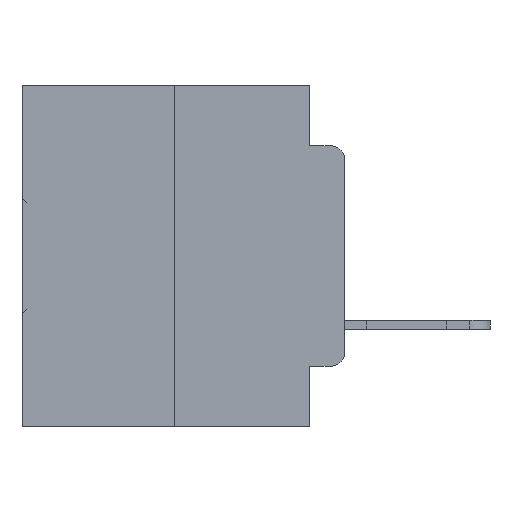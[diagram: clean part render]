
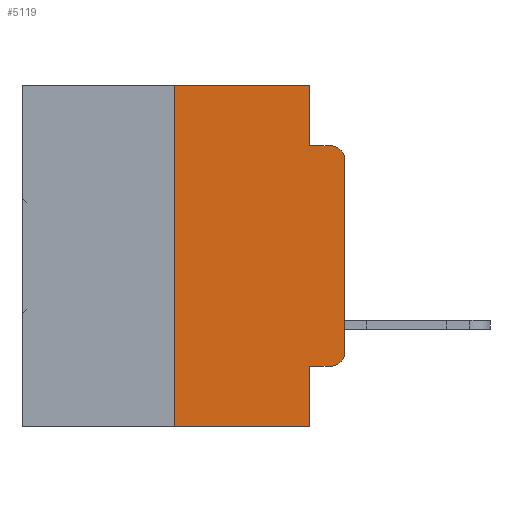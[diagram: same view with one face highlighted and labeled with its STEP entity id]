
A CAD part, left-side view. The second image highlights one B-rep face of the part: STEP entity #5119.
In plain terms, the highlighted planar face has unit normal (-1, 0, 0).
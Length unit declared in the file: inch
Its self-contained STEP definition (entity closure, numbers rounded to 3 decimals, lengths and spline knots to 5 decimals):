
#803 = EDGE_CURVE ( 'NONE', #9963, #8010, #15396, .T. ) ;
#901 = LINE ( 'NONE', #18941, #27302 ) ;
#1038 = VECTOR ( 'NONE', #20745, 39.37008 ) ;
#1166 = CARTESIAN_POINT ( 'NONE',  ( 0., 0.02, -0.1085 ) ) ;
#1177 = ORIENTED_EDGE ( 'NONE', *, *, #20023, .F. ) ;
#1184 = LINE ( 'NONE', #7125, #21236 ) ;
#1892 = ORIENTED_EDGE ( 'NONE', *, *, #803, .T. ) ;
#1928 = DIRECTION ( 'NONE',  ( 0., 0., 1. ) ) ;
#2142 = VECTOR ( 'NONE', #24793, 39.37008 ) ;
#2154 = CARTESIAN_POINT ( 'NONE',  ( 0., 0.25, 0. ) ) ;
#3332 = ORIENTED_EDGE ( 'NONE', *, *, #16567, .T. ) ;
#3963 = DIRECTION ( 'NONE',  ( 0., 0., -1. ) ) ;
#5119 = ADVANCED_FACE ( 'NONE', ( #9822 ), #17252, .F. ) ;
#5909 = EDGE_CURVE ( 'NONE', #9963, #8223, #8118, .T. ) ;
#5964 = DIRECTION ( 'NONE',  ( 0., -1., 0. ) ) ;
#6151 = CARTESIAN_POINT ( 'NONE',  ( 0., 0.051, -0.0885 ) ) ;
#6654 = CARTESIAN_POINT ( 'NONE',  ( 0., 0.051, -0.4115 ) ) ;
#6997 = VERTEX_POINT ( 'NONE', #6151 ) ;
#7125 = CARTESIAN_POINT ( 'NONE',  ( 0., 0., 0. ) ) ;
#7772 = EDGE_CURVE ( 'NONE', #25397, #6997, #9429, .T. ) ;
#8010 = VERTEX_POINT ( 'NONE', #17255 ) ;
#8118 = LINE ( 'NONE', #2154, #20095 ) ;
#8223 = VERTEX_POINT ( 'NONE', #30331 ) ;
#8350 = CARTESIAN_POINT ( 'NONE',  ( 0., 0.02, -0.3915 ) ) ;
#9429 = LINE ( 'NONE', #24865, #2142 ) ;
#9511 = VERTEX_POINT ( 'NONE', #28037 ) ;
#9822 = FACE_OUTER_BOUND ( 'NONE', #19943, .T. ) ;
#9963 = VERTEX_POINT ( 'NONE', #30104 ) ;
#10439 = ORIENTED_EDGE ( 'NONE', *, *, #29847, .F. ) ;
#10693 = AXIS2_PLACEMENT_3D ( 'NONE', #1166, #19587, #3963 ) ;
#10838 = ORIENTED_EDGE ( 'NONE', *, *, #18798, .T. ) ;
#11002 = DIRECTION ( 'NONE',  ( 0., 0., -1. ) ) ;
#12067 = DIRECTION ( 'NONE',  ( 0., 0., -1. ) ) ;
#13087 = EDGE_CURVE ( 'NONE', #6997, #22821, #901, .T. ) ;
#13448 = VECTOR ( 'NONE', #12067, 39.37008 ) ;
#13790 = LINE ( 'NONE', #31032, #25941 ) ;
#14772 = CIRCLE ( 'NONE', #23573, 0.02 ) ;
#15396 = LINE ( 'NONE', #21263, #1038 ) ;
#15498 = EDGE_CURVE ( 'NONE', #23687, #9511, #14772, .T. ) ;
#15734 = ORIENTED_EDGE ( 'NONE', *, *, #18191, .T. ) ;
#16567 = EDGE_CURVE ( 'NONE', #26871, #22821, #30393, .T. ) ;
#17109 = DIRECTION ( 'NONE',  ( 0., 0., -1. ) ) ;
#17145 = DIRECTION ( 'NONE',  ( 1., 0., 0. ) ) ;
#17214 = CARTESIAN_POINT ( 'NONE',  ( 0., 0.473, 0. ) ) ;
#17252 = PLANE ( 'NONE',  #29375 ) ;
#17255 = CARTESIAN_POINT ( 'NONE',  ( 0., 0.051, -0.5 ) ) ;
#18191 = EDGE_CURVE ( 'NONE', #9511, #26871, #1184, .T. ) ;
#18798 = EDGE_CURVE ( 'NONE', #32650, #23687, #27502, .T. ) ;
#18941 = CARTESIAN_POINT ( 'NONE',  ( 0., 0.051, -0.0885 ) ) ;
#19566 = CARTESIAN_POINT ( 'NONE',  ( 0., 0.051, 0. ) ) ;
#19587 = DIRECTION ( 'NONE',  ( -1., 0., 0. ) ) ;
#19943 = EDGE_LOOP ( 'NONE', ( #15734, #3332, #25628, #23700, #1177, #28460, #1892, #10439, #10838, #24055 ) ) ;
#20023 = EDGE_CURVE ( 'NONE', #8223, #25397, #13790, .T. ) ;
#20095 = VECTOR ( 'NONE', #1928, 39.37008 ) ;
#20745 = DIRECTION ( 'NONE',  ( 0., -1., 0. ) ) ;
#21236 = VECTOR ( 'NONE', #22315, 39.37008 ) ;
#21263 = CARTESIAN_POINT ( 'NONE',  ( 0., 0.473, -0.5 ) ) ;
#22315 = DIRECTION ( 'NONE',  ( 0., 0., 1. ) ) ;
#22821 = VERTEX_POINT ( 'NONE', #23223 ) ;
#23223 = CARTESIAN_POINT ( 'NONE',  ( 0., 0.02, -0.0885 ) ) ;
#23573 = AXIS2_PLACEMENT_3D ( 'NONE', #8350, #25757, #11002 ) ;
#23687 = VERTEX_POINT ( 'NONE', #30467 ) ;
#23700 = ORIENTED_EDGE ( 'NONE', *, *, #7772, .F. ) ;
#23974 = CARTESIAN_POINT ( 'NONE',  ( 0., 0.051, -0.4115 ) ) ;
#24055 = ORIENTED_EDGE ( 'NONE', *, *, #15498, .T. ) ;
#24103 = DIRECTION ( 'NONE',  ( 0., -1., 0. ) ) ;
#24254 = CARTESIAN_POINT ( 'NONE',  ( 0., 0.051, 0. ) ) ;
#24476 = CARTESIAN_POINT ( 'NONE',  ( 0., 0., -0.1085 ) ) ;
#24793 = DIRECTION ( 'NONE',  ( 0., 0., -1. ) ) ;
#24865 = CARTESIAN_POINT ( 'NONE',  ( 0., 0.051, 0. ) ) ;
#25397 = VERTEX_POINT ( 'NONE', #24254 ) ;
#25628 = ORIENTED_EDGE ( 'NONE', *, *, #13087, .F. ) ;
#25757 = DIRECTION ( 'NONE',  ( -1., 0., 0. ) ) ;
#25941 = VECTOR ( 'NONE', #24103, 39.37008 ) ;
#26359 = DIRECTION ( 'NONE',  ( 0., -1., 0. ) ) ;
#26386 = LINE ( 'NONE', #19566, #13448 ) ;
#26741 = VECTOR ( 'NONE', #26359, 39.37008 ) ;
#26871 = VERTEX_POINT ( 'NONE', #24476 ) ;
#27302 = VECTOR ( 'NONE', #5964, 39.37008 ) ;
#27502 = LINE ( 'NONE', #23974, #26741 ) ;
#28037 = CARTESIAN_POINT ( 'NONE',  ( 0., 0., -0.3915 ) ) ;
#28460 = ORIENTED_EDGE ( 'NONE', *, *, #5909, .F. ) ;
#29375 = AXIS2_PLACEMENT_3D ( 'NONE', #17214, #17145, #17109 ) ;
#29847 = EDGE_CURVE ( 'NONE', #32650, #8010, #26386, .T. ) ;
#30104 = CARTESIAN_POINT ( 'NONE',  ( 0., 0.25, -0.5 ) ) ;
#30331 = CARTESIAN_POINT ( 'NONE',  ( 0., 0.25, 0. ) ) ;
#30393 = CIRCLE ( 'NONE', #10693, 0.02 ) ;
#30467 = CARTESIAN_POINT ( 'NONE',  ( 0., 0.02, -0.4115 ) ) ;
#31032 = CARTESIAN_POINT ( 'NONE',  ( 0., 0.473, 0. ) ) ;
#32650 = VERTEX_POINT ( 'NONE', #6654 ) ;
